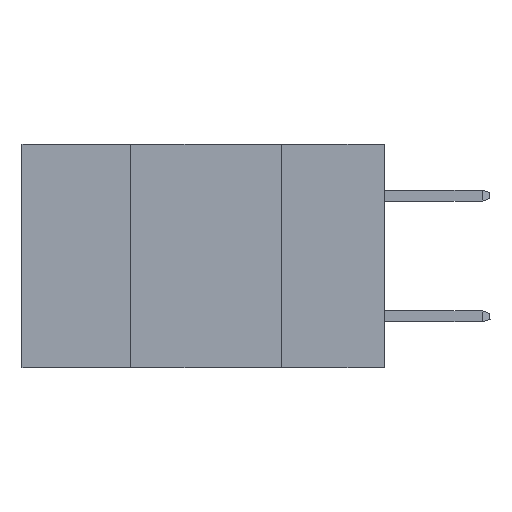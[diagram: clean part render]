
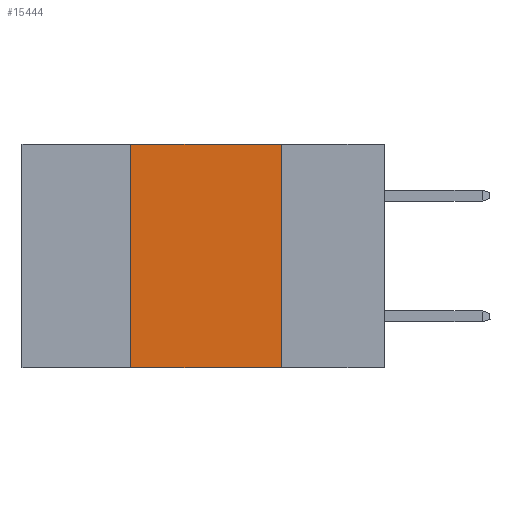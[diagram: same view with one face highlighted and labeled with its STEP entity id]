
A CAD part, left-side view. The second image highlights one B-rep face of the part: STEP entity #15444.
In plain terms, the highlighted planar face has unit normal (-1, 0, 0).
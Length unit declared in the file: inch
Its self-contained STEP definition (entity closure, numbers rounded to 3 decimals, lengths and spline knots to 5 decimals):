
#474 = CARTESIAN_POINT ( 'NONE',  ( 0., 0.17, 0. ) ) ;
#1460 = PLANE ( 'NONE',  #4340 ) ;
#1725 = DIRECTION ( 'NONE',  ( 0., 0., -1. ) ) ;
#3223 = ORIENTED_EDGE ( 'NONE', *, *, #21920, .F. ) ;
#4328 = LINE ( 'NONE', #6557, #9479 ) ;
#4340 = AXIS2_PLACEMENT_3D ( 'NONE', #23972, #9140, #26408 ) ;
#4695 = VERTEX_POINT ( 'NONE', #474 ) ;
#5181 = VECTOR ( 'NONE', #11552, 39.37008 ) ;
#6557 = CARTESIAN_POINT ( 'NONE',  ( 0., 0.42, 0. ) ) ;
#6705 = EDGE_CURVE ( 'NONE', #14535, #31276, #7199, .T. ) ;
#7199 = LINE ( 'NONE', #26063, #13117 ) ;
#9057 = FACE_OUTER_BOUND ( 'NONE', #30802, .T. ) ;
#9140 = DIRECTION ( 'NONE',  ( 1., 0., 0. ) ) ;
#9479 = VECTOR ( 'NONE', #14138, 39.37008 ) ;
#9731 = CARTESIAN_POINT ( 'NONE',  ( 0., 0.42, -0.37 ) ) ;
#9894 = CARTESIAN_POINT ( 'NONE',  ( 0., 0.42, 0. ) ) ;
#9964 = ORIENTED_EDGE ( 'NONE', *, *, #12946, .F. ) ;
#11552 = DIRECTION ( 'NONE',  ( 0., -1., 0. ) ) ;
#11866 = LINE ( 'NONE', #16440, #5181 ) ;
#12304 = ORIENTED_EDGE ( 'NONE', *, *, #6705, .T. ) ;
#12946 = EDGE_CURVE ( 'NONE', #19068, #4695, #11866, .T. ) ;
#13117 = VECTOR ( 'NONE', #13791, 39.37008 ) ;
#13638 = EDGE_CURVE ( 'NONE', #14535, #19068, #4328, .T. ) ;
#13791 = DIRECTION ( 'NONE',  ( 0., -1., 0. ) ) ;
#14138 = DIRECTION ( 'NONE',  ( 0., 0., 1. ) ) ;
#14535 = VERTEX_POINT ( 'NONE', #9731 ) ;
#15444 = ADVANCED_FACE ( 'NONE', ( #9057 ), #1460, .F. ) ;
#16440 = CARTESIAN_POINT ( 'NONE',  ( 0., 0.6, 0. ) ) ;
#18405 = LINE ( 'NONE', #19411, #24171 ) ;
#19068 = VERTEX_POINT ( 'NONE', #9894 ) ;
#19411 = CARTESIAN_POINT ( 'NONE',  ( 0., 0.17, 0. ) ) ;
#21920 = EDGE_CURVE ( 'NONE', #4695, #31276, #18405, .T. ) ;
#23895 = ORIENTED_EDGE ( 'NONE', *, *, #13638, .F. ) ;
#23972 = CARTESIAN_POINT ( 'NONE',  ( 0., 0.6, 0. ) ) ;
#24171 = VECTOR ( 'NONE', #1725, 39.37008 ) ;
#26063 = CARTESIAN_POINT ( 'NONE',  ( 0., 0.6, -0.37 ) ) ;
#26408 = DIRECTION ( 'NONE',  ( 0., 0., -1. ) ) ;
#30717 = CARTESIAN_POINT ( 'NONE',  ( 0., 0.17, -0.37 ) ) ;
#30802 = EDGE_LOOP ( 'NONE', ( #3223, #9964, #23895, #12304 ) ) ;
#31276 = VERTEX_POINT ( 'NONE', #30717 ) ;
